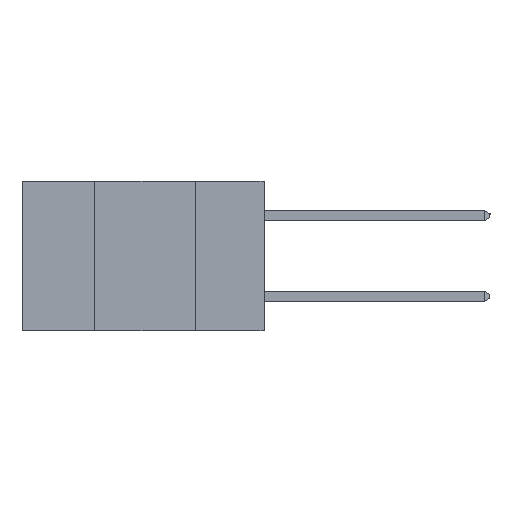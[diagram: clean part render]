
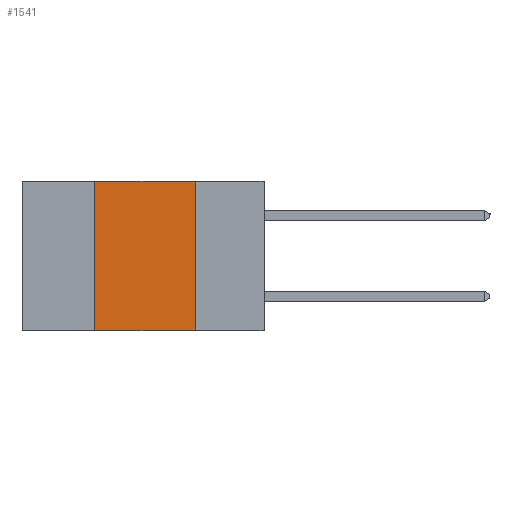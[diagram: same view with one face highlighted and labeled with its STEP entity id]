
A CAD part, left-side view. The second image highlights one B-rep face of the part: STEP entity #1541.
In plain terms, the highlighted planar face has unit normal (-1, 0, 0).
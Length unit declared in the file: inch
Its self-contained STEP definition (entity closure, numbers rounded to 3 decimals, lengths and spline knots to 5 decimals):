
#525 = CARTESIAN_POINT ( 'NONE',  ( 0., 0.6, 0. ) ) ;
#925 = ORIENTED_EDGE ( 'NONE', *, *, #23305, .F. ) ;
#1541 = ADVANCED_FACE ( 'NONE', ( #2705 ), #18242, .F. ) ;
#1564 = VECTOR ( 'NONE', #20967, 39.37008 ) ;
#2253 = VECTOR ( 'NONE', #8853, 39.37008 ) ;
#2374 = VECTOR ( 'NONE', #12047, 39.37008 ) ;
#2383 = LINE ( 'NONE', #10390, #2374 ) ;
#2492 = CARTESIAN_POINT ( 'NONE',  ( 0., 0.6, -0.37 ) ) ;
#2705 = FACE_OUTER_BOUND ( 'NONE', #9441, .T. ) ;
#3044 = DIRECTION ( 'NONE',  ( 0., -1., 0. ) ) ;
#3893 = VERTEX_POINT ( 'NONE', #20736 ) ;
#5451 = CARTESIAN_POINT ( 'NONE',  ( 0., 0.17, 0. ) ) ;
#8853 = DIRECTION ( 'NONE',  ( 0., -1., 0. ) ) ;
#9441 = EDGE_LOOP ( 'NONE', ( #925, #21591, #21081, #10378 ) ) ;
#10260 = VERTEX_POINT ( 'NONE', #14585 ) ;
#10378 = ORIENTED_EDGE ( 'NONE', *, *, #13347, .T. ) ;
#10390 = CARTESIAN_POINT ( 'NONE',  ( 0., 0.17, -0.37 ) ) ;
#11971 = VECTOR ( 'NONE', #3044, 39.37008 ) ;
#12047 = DIRECTION ( 'NONE',  ( 0., 0., -1. ) ) ;
#12724 = CARTESIAN_POINT ( 'NONE',  ( 0., 0.6, 0. ) ) ;
#13011 = AXIS2_PLACEMENT_3D ( 'NONE', #525, #15942, #14026 ) ;
#13347 = EDGE_CURVE ( 'NONE', #3893, #18835, #22468, .T. ) ;
#14026 = DIRECTION ( 'NONE',  ( 0., 0., -1. ) ) ;
#14585 = CARTESIAN_POINT ( 'NONE',  ( 0., 0.42, 0. ) ) ;
#15239 = CARTESIAN_POINT ( 'NONE',  ( 0., 0.42, -0.37 ) ) ;
#15942 = DIRECTION ( 'NONE',  ( 1., 0., 0. ) ) ;
#17390 = EDGE_CURVE ( 'NONE', #3893, #10260, #21101, .T. ) ;
#18242 = PLANE ( 'NONE',  #13011 ) ;
#18659 = EDGE_CURVE ( 'NONE', #10260, #24952, #22648, .T. ) ;
#18835 = VERTEX_POINT ( 'NONE', #23014 ) ;
#20736 = CARTESIAN_POINT ( 'NONE',  ( 0., 0.42, -0.37 ) ) ;
#20967 = DIRECTION ( 'NONE',  ( 0., 0., 1. ) ) ;
#21081 = ORIENTED_EDGE ( 'NONE', *, *, #17390, .F. ) ;
#21101 = LINE ( 'NONE', #15239, #1564 ) ;
#21591 = ORIENTED_EDGE ( 'NONE', *, *, #18659, .F. ) ;
#22468 = LINE ( 'NONE', #2492, #2253 ) ;
#22648 = LINE ( 'NONE', #12724, #11971 ) ;
#23014 = CARTESIAN_POINT ( 'NONE',  ( 0., 0.17, -0.37 ) ) ;
#23305 = EDGE_CURVE ( 'NONE', #24952, #18835, #2383, .T. ) ;
#24952 = VERTEX_POINT ( 'NONE', #5451 ) ;
